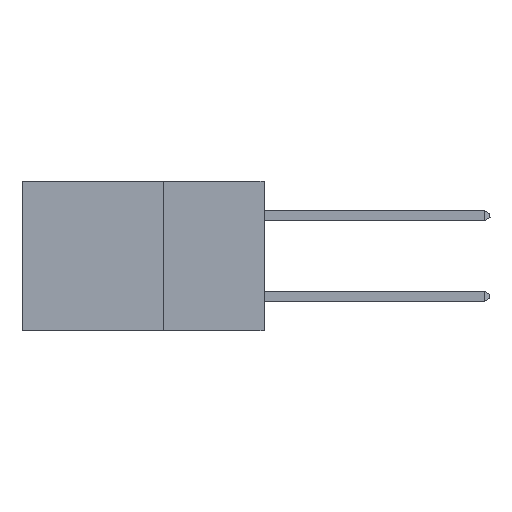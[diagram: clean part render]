
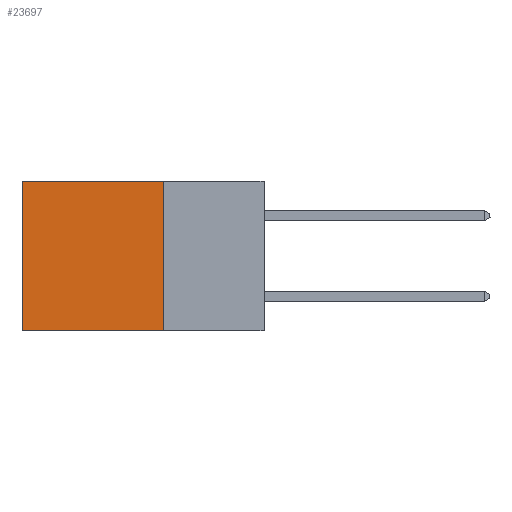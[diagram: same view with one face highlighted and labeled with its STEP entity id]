
A CAD part, left-side view. The second image highlights one B-rep face of the part: STEP entity #23697.
In plain terms, the highlighted planar face has unit normal (-1, 0, 0).
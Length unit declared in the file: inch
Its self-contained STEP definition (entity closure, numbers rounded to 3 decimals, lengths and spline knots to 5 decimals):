
#454 = EDGE_LOOP ( 'NONE', ( #979, #7676, #18726, #2659 ) ) ;
#979 = ORIENTED_EDGE ( 'NONE', *, *, #13875, .T. ) ;
#2199 = DIRECTION ( 'NONE',  ( 0., 0., -1. ) ) ;
#2316 = LINE ( 'NONE', #21450, #3288 ) ;
#2372 = DIRECTION ( 'NONE',  ( 0., 0., -1. ) ) ;
#2659 = ORIENTED_EDGE ( 'NONE', *, *, #12277, .T. ) ;
#3288 = VECTOR ( 'NONE', #9341, 39.37008 ) ;
#3785 = LINE ( 'NONE', #13095, #18634 ) ;
#4317 = VECTOR ( 'NONE', #17519, 39.37008 ) ;
#4371 = VERTEX_POINT ( 'NONE', #15743 ) ;
#4891 = CARTESIAN_POINT ( 'NONE',  ( 0.298, 0.25, -0.37 ) ) ;
#5868 = CARTESIAN_POINT ( 'NONE',  ( 0.298, 0.6, -0.37 ) ) ;
#6149 = CARTESIAN_POINT ( 'NONE',  ( 0.298, 0.25, 0. ) ) ;
#6810 = VERTEX_POINT ( 'NONE', #20062 ) ;
#7676 = ORIENTED_EDGE ( 'NONE', *, *, #7940, .F. ) ;
#7940 = EDGE_CURVE ( 'NONE', #4371, #19337, #17520, .T. ) ;
#8852 = VERTEX_POINT ( 'NONE', #21607 ) ;
#9341 = DIRECTION ( 'NONE',  ( 0., 1., 0. ) ) ;
#12277 = EDGE_CURVE ( 'NONE', #8852, #6810, #2316, .T. ) ;
#13095 = CARTESIAN_POINT ( 'NONE',  ( 0.298, 0.6, 0. ) ) ;
#13875 = EDGE_CURVE ( 'NONE', #6810, #19337, #3785, .T. ) ;
#14256 = DIRECTION ( 'NONE',  ( 1., 0., 0. ) ) ;
#15242 = LINE ( 'NONE', #24876, #21028 ) ;
#15743 = CARTESIAN_POINT ( 'NONE',  ( 0.298, 0.25, -0.37 ) ) ;
#16158 = AXIS2_PLACEMENT_3D ( 'NONE', #6149, #14256, #2199 ) ;
#17519 = DIRECTION ( 'NONE',  ( 0., 1., 0. ) ) ;
#17520 = LINE ( 'NONE', #4891, #4317 ) ;
#18634 = VECTOR ( 'NONE', #21014, 39.37008 ) ;
#18726 = ORIENTED_EDGE ( 'NONE', *, *, #21680, .F. ) ;
#19337 = VERTEX_POINT ( 'NONE', #5868 ) ;
#20062 = CARTESIAN_POINT ( 'NONE',  ( 0.298, 0.6, 0. ) ) ;
#20618 = FACE_OUTER_BOUND ( 'NONE', #454, .T. ) ;
#21014 = DIRECTION ( 'NONE',  ( 0., 0., -1. ) ) ;
#21028 = VECTOR ( 'NONE', #2372, 39.37008 ) ;
#21450 = CARTESIAN_POINT ( 'NONE',  ( 0.298, 0.25, 0. ) ) ;
#21607 = CARTESIAN_POINT ( 'NONE',  ( 0.298, 0.25, 0. ) ) ;
#21680 = EDGE_CURVE ( 'NONE', #8852, #4371, #15242, .T. ) ;
#23697 = ADVANCED_FACE ( 'NONE', ( #20618 ), #26591, .F. ) ;
#24876 = CARTESIAN_POINT ( 'NONE',  ( 0.298, 0.25, 0. ) ) ;
#26591 = PLANE ( 'NONE',  #16158 ) ;
